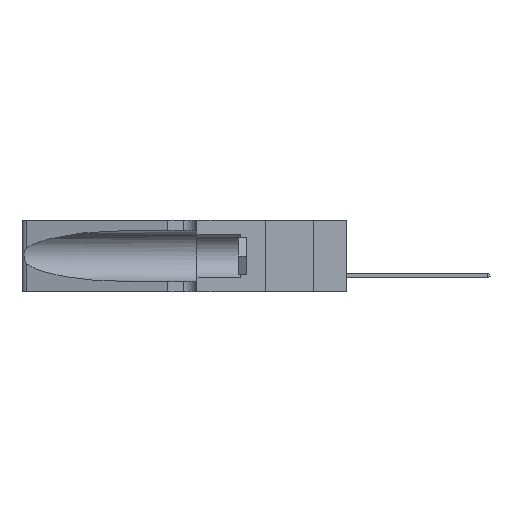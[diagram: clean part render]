
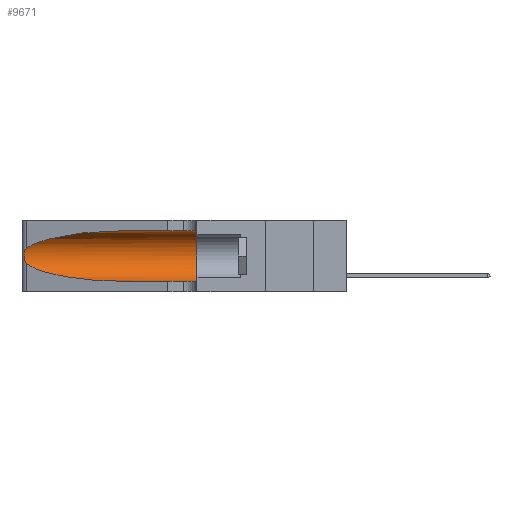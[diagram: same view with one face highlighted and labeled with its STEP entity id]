
A CAD part, left-side view. The second image highlights one B-rep face of the part: STEP entity #9671.
In plain terms, the highlighted cylindrical face has radius 3.308 mm (diameter 6.617 mm), a partial arc.
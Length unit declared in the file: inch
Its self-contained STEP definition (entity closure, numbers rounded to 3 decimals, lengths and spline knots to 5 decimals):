
#858 = DIRECTION ( 'NONE',  ( 0., 1., 0. ) ) ;
#1222 = EDGE_CURVE ( 'NONE', #10814, #31547, #19709, .T. ) ;
#1649 = ORIENTED_EDGE ( 'NONE', *, *, #5397, .F. ) ;
#2654 = CARTESIAN_POINT ( 'NONE',  ( 0.26075, 1.23896, 0.178 ) ) ;
#2933 = CARTESIAN_POINT ( 'NONE',  ( 0.2373, 1.15595, 0.28018 ) ) ;
#5382 = CARTESIAN_POINT ( 'NONE',  ( 0.26017, 1.23833, 0.17102 ) ) ;
#5397 = EDGE_CURVE ( 'NONE', #29975, #5514, #6868, .T. ) ;
#5502 = CARTESIAN_POINT ( 'NONE',  ( 0.25856, 1.23593, 0.16098 ) ) ;
#5514 = VERTEX_POINT ( 'NONE', #27857 ) ;
#5685 = CARTESIAN_POINT ( 'NONE',  ( 0.25487, 1.22718, 0.22369 ) ) ;
#6162 = CARTESIAN_POINT ( 'NONE',  ( 0.1305, 0.72297, 0.05475 ) ) ;
#6868 = LINE ( 'NONE', #23739, #28932 ) ;
#7040 = DIRECTION ( 'NONE',  ( 0., -1., 0. ) ) ;
#7544 = DIRECTION ( 'NONE',  ( 0., -1., 0. ) ) ;
#7663 = CARTESIAN_POINT ( 'NONE',  ( 0.1305, 0.72297, 0.31525 ) ) ;
#8434 = ORIENTED_EDGE ( 'NONE', *, *, #29604, .T. ) ;
#9241 = CARTESIAN_POINT ( 'NONE',  ( 0.25787, 1.23484, 0.2124 ) ) ;
#9671 = ADVANCED_FACE ( 'NONE', ( #28725 ), #21364, .F. ) ;
#10814 = VERTEX_POINT ( 'NONE', #6162 ) ;
#12356 = CARTESIAN_POINT ( 'NONE',  ( 0.1305, 0.72297, 0.05475 ) ) ;
#12794 = CARTESIAN_POINT ( 'NONE',  ( 0.25639, 1.23184, 0.21858 ) ) ;
#12798 = B_SPLINE_CURVE_WITH_KNOTS ( 'NONE', 3,
 ( #24930, #33073, #12794, #9241, #28567, #31678, #15664, #2654, #5382, #5502, #28679, #23322, #21014, #26259 ),
 .UNSPECIFIED., .F., .F.,
 ( 4, 2, 2, 2, 2, 2, 4 ),
 ( 0., 0.00027, 0.00053, 0.00107, 0.0016, 0.00187, 0.00214 ),
 .UNSPECIFIED. ) ;
#13012 = CARTESIAN_POINT ( 'NONE',  ( 0.1305, 1.61858, 0.05475 ) ) ;
#13987 = CARTESIAN_POINT ( 'NONE',  ( 0.25487, 1.22718, 0.14631 ) ) ;
#14974 = VERTEX_POINT ( 'NONE', #13987 ) ;
#15664 = CARTESIAN_POINT ( 'NONE',  ( 0.26075, 1.23896, 0.19203 ) ) ;
#15665 = CARTESIAN_POINT ( 'NONE',  ( 0.1305, 0.35, 0.05475 ) ) ;
#17201 = CARTESIAN_POINT ( 'NONE',  ( 0.25487, 1.22718, 0.22369 ) ) ;
#17518 = CARTESIAN_POINT ( 'NONE',  ( 0.25487, 1.22718, 0.14631 ) ) ;
#17854 = CARTESIAN_POINT ( 'NONE',  ( 0.2373, 1.15595, 0.08982 ) ) ;
#17948 = VERTEX_POINT ( 'NONE', #17201 ) ;
#18448 =( BOUNDED_CURVE ( )  B_SPLINE_CURVE ( 3, ( #31643, #18579, #2933, #5685 ),
 .UNSPECIFIED., .F., .T. ) 
 B_SPLINE_CURVE_WITH_KNOTS ( ( 4, 4 ),
 ( 1.5708, 2.84003 ),
 .UNSPECIFIED. ) 
 CURVE ( )  GEOMETRIC_REPRESENTATION_ITEM ( )  RATIONAL_B_SPLINE_CURVE ( ( 1., 0.87, 0.87, 1. ) ) 
 REPRESENTATION_ITEM ( '' )  );
#18579 = CARTESIAN_POINT ( 'NONE',  ( 0.18966, 0.96281, 0.31525 ) ) ;
#19163 = DIRECTION ( 'NONE',  ( 0., 0., 1. ) ) ;
#19321 = VECTOR ( 'NONE', #7544, 39.37008 ) ;
#19397 = CIRCLE ( 'NONE', #22413, 0.13025 ) ;
#19709 = LINE ( 'NONE', #13012, #19321 ) ;
#21014 = CARTESIAN_POINT ( 'NONE',  ( 0.25555, 1.22993, 0.14849 ) ) ;
#21364 = CYLINDRICAL_SURFACE ( 'NONE', #28069, 0.13025 ) ;
#21886 = EDGE_CURVE ( 'NONE', #14974, #10814, #32972, .T. ) ;
#22044 = ORIENTED_EDGE ( 'NONE', *, *, #1222, .T. ) ;
#22325 = ORIENTED_EDGE ( 'NONE', *, *, #27169, .T. ) ;
#22413 = AXIS2_PLACEMENT_3D ( 'NONE', #29771, #858, #19163 ) ;
#22555 = EDGE_CURVE ( 'NONE', #5514, #31547, #19397, .T. ) ;
#23180 = ORIENTED_EDGE ( 'NONE', *, *, #22555, .F. ) ;
#23322 = CARTESIAN_POINT ( 'NONE',  ( 0.25639, 1.23186, 0.15144 ) ) ;
#23739 = CARTESIAN_POINT ( 'NONE',  ( 0.1305, 1.61858, 0.31525 ) ) ;
#24082 = DIRECTION ( 'NONE',  ( 0., -1., 0. ) ) ;
#24930 = CARTESIAN_POINT ( 'NONE',  ( 0.25487, 1.22718, 0.22369 ) ) ;
#25463 = DIRECTION ( 'NONE',  ( 0., 0., -1. ) ) ;
#26259 = CARTESIAN_POINT ( 'NONE',  ( 0.25487, 1.22718, 0.14631 ) ) ;
#26284 = ORIENTED_EDGE ( 'NONE', *, *, #21886, .T. ) ;
#27169 = EDGE_CURVE ( 'NONE', #17948, #14974, #12798, .T. ) ;
#27857 = CARTESIAN_POINT ( 'NONE',  ( 0.1305, 0.35, 0.31525 ) ) ;
#28069 = AXIS2_PLACEMENT_3D ( 'NONE', #30607, #7040, #25463 ) ;
#28232 = CARTESIAN_POINT ( 'NONE',  ( 0.18966, 0.96281, 0.05475 ) ) ;
#28567 = CARTESIAN_POINT ( 'NONE',  ( 0.25854, 1.2359, 0.20912 ) ) ;
#28679 = CARTESIAN_POINT ( 'NONE',  ( 0.25789, 1.23486, 0.15765 ) ) ;
#28725 = FACE_OUTER_BOUND ( 'NONE', #31728, .T. ) ;
#28932 = VECTOR ( 'NONE', #24082, 39.37008 ) ;
#29604 = EDGE_CURVE ( 'NONE', #29975, #17948, #18448, .T. ) ;
#29771 = CARTESIAN_POINT ( 'NONE',  ( 0.1305, 0.35, 0.185 ) ) ;
#29975 = VERTEX_POINT ( 'NONE', #7663 ) ;
#30607 = CARTESIAN_POINT ( 'NONE',  ( 0.1305, 1.61858, 0.185 ) ) ;
#31547 = VERTEX_POINT ( 'NONE', #15665 ) ;
#31643 = CARTESIAN_POINT ( 'NONE',  ( 0.1305, 0.72297, 0.31525 ) ) ;
#31678 = CARTESIAN_POINT ( 'NONE',  ( 0.26018, 1.23835, 0.19895 ) ) ;
#31728 = EDGE_LOOP ( 'NONE', ( #8434, #22325, #26284, #22044, #23180, #1649 ) ) ;
#32972 =( BOUNDED_CURVE ( )  B_SPLINE_CURVE ( 3, ( #17518, #17854, #28232, #12356 ),
 .UNSPECIFIED., .F., .F. ) 
 B_SPLINE_CURVE_WITH_KNOTS ( ( 4, 4 ),
 ( 3.44316, 4.71239 ),
 .UNSPECIFIED. ) 
 CURVE ( )  GEOMETRIC_REPRESENTATION_ITEM ( )  RATIONAL_B_SPLINE_CURVE ( ( 1., 0.87, 0.87, 1. ) ) 
 REPRESENTATION_ITEM ( '' )  );
#33073 = CARTESIAN_POINT ( 'NONE',  ( 0.25555, 1.22994, 0.2215 ) ) ;
